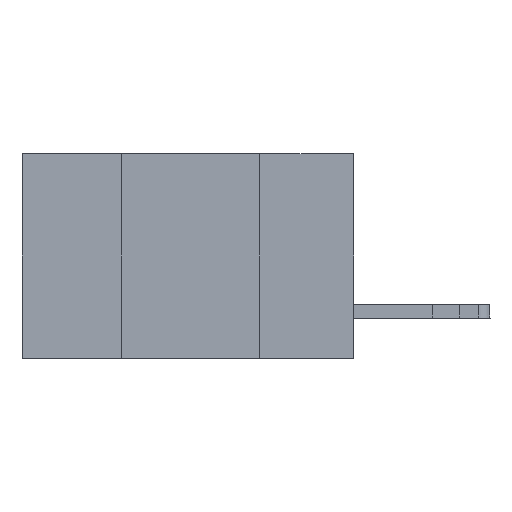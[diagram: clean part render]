
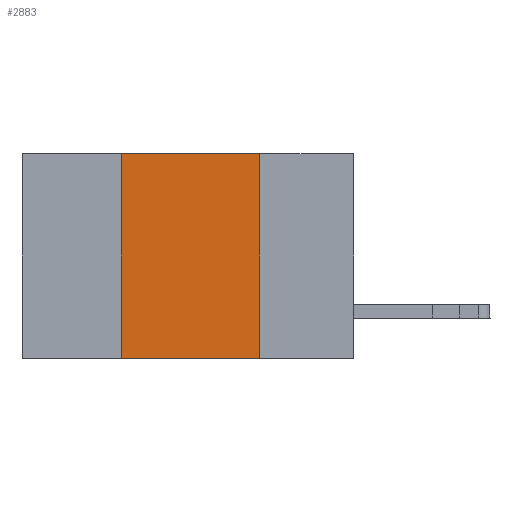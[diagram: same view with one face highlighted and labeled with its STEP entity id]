
A CAD part, left-side view. The second image highlights one B-rep face of the part: STEP entity #2883.
In plain terms, the highlighted planar face has unit normal (-1, 0, 0).
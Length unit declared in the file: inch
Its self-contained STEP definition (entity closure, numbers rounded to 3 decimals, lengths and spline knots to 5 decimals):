
#421 = EDGE_CURVE ( 'NONE', #19738, #24610, #35424, .T. ) ;
#920 = VERTEX_POINT ( 'NONE', #13419 ) ;
#1744 = VECTOR ( 'NONE', #30529, 39.37008 ) ;
#2042 = DIRECTION ( 'NONE',  ( 0., -1., 0. ) ) ;
#2181 = CARTESIAN_POINT ( 'NONE',  ( 0., 0.6, 0. ) ) ;
#2883 = ADVANCED_FACE ( 'NONE', ( #23632 ), #18873, .F. ) ;
#4973 = DIRECTION ( 'NONE',  ( 1., 0., 0. ) ) ;
#6508 = VECTOR ( 'NONE', #21416, 39.37008 ) ;
#9399 = EDGE_CURVE ( 'NONE', #920, #19738, #23984, .T. ) ;
#9880 = EDGE_CURVE ( 'NONE', #19774, #920, #35956, .T. ) ;
#10194 = CARTESIAN_POINT ( 'NONE',  ( 0., 0.42, 0. ) ) ;
#10302 = CARTESIAN_POINT ( 'NONE',  ( 0., 0.6, -0.37 ) ) ;
#13000 = LINE ( 'NONE', #10302, #19526 ) ;
#13075 = CARTESIAN_POINT ( 'NONE',  ( 0., 0.17, -0.37 ) ) ;
#13155 = EDGE_LOOP ( 'NONE', ( #24995, #17600, #20027, #23932 ) ) ;
#13419 = CARTESIAN_POINT ( 'NONE',  ( 0., 0.42, 0. ) ) ;
#14074 = CARTESIAN_POINT ( 'NONE',  ( 0., 0.17, 0. ) ) ;
#17600 = ORIENTED_EDGE ( 'NONE', *, *, #9399, .F. ) ;
#18873 = PLANE ( 'NONE',  #30373 ) ;
#19526 = VECTOR ( 'NONE', #2042, 39.37008 ) ;
#19738 = VERTEX_POINT ( 'NONE', #32236 ) ;
#19774 = VERTEX_POINT ( 'NONE', #26950 ) ;
#20027 = ORIENTED_EDGE ( 'NONE', *, *, #9880, .F. ) ;
#21416 = DIRECTION ( 'NONE',  ( 0., 0., 1. ) ) ;
#22259 = EDGE_CURVE ( 'NONE', #19774, #24610, #13000, .T. ) ;
#23632 = FACE_OUTER_BOUND ( 'NONE', #13155, .T. ) ;
#23932 = ORIENTED_EDGE ( 'NONE', *, *, #22259, .T. ) ;
#23984 = LINE ( 'NONE', #27743, #1744 ) ;
#24474 = DIRECTION ( 'NONE',  ( 0., 0., -1. ) ) ;
#24610 = VERTEX_POINT ( 'NONE', #13075 ) ;
#24995 = ORIENTED_EDGE ( 'NONE', *, *, #421, .F. ) ;
#26950 = CARTESIAN_POINT ( 'NONE',  ( 0., 0.42, -0.37 ) ) ;
#27743 = CARTESIAN_POINT ( 'NONE',  ( 0., 0.6, 0. ) ) ;
#30373 = AXIS2_PLACEMENT_3D ( 'NONE', #2181, #4973, #24474 ) ;
#30529 = DIRECTION ( 'NONE',  ( 0., -1., 0. ) ) ;
#30649 = DIRECTION ( 'NONE',  ( 0., 0., -1. ) ) ;
#32236 = CARTESIAN_POINT ( 'NONE',  ( 0., 0.17, 0. ) ) ;
#34578 = VECTOR ( 'NONE', #30649, 39.37008 ) ;
#35424 = LINE ( 'NONE', #14074, #34578 ) ;
#35956 = LINE ( 'NONE', #10194, #6508 ) ;
